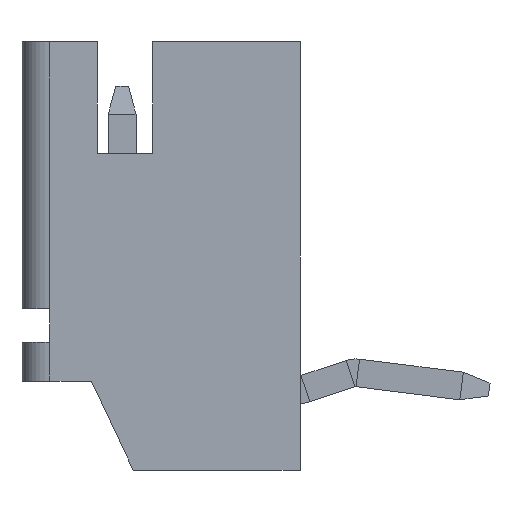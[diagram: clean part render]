
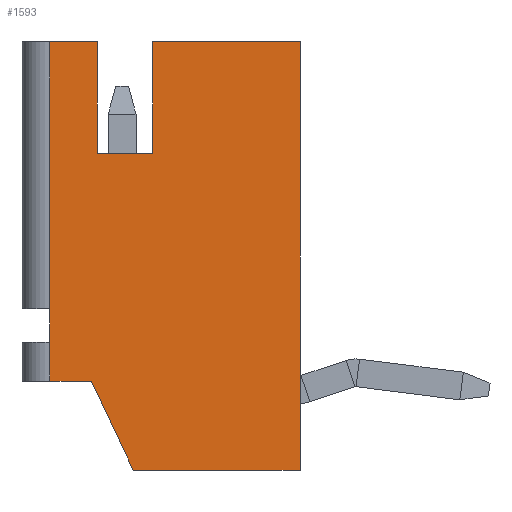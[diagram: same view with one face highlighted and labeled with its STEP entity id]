
A CAD part, left-side view. The second image highlights one B-rep face of the part: STEP entity #1593.
In plain terms, the highlighted planar face has unit normal (-1, 0, 0).
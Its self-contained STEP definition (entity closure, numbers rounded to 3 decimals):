
#33 = VERTEX_POINT ( 'NONE', #2794 ) ;
#44 = DIRECTION ( 'NONE',  ( 0., 0., -1. ) ) ;
#70 = EDGE_CURVE ( 'NONE', #2506, #1294, #556, .T. ) ;
#76 = VERTEX_POINT ( 'NONE', #2383 ) ;
#103 = CARTESIAN_POINT ( 'NONE',  ( -2., -3.2, 6.1 ) ) ;
#114 = LINE ( 'NONE', #1688, #1671 ) ;
#117 = DIRECTION ( 'NONE',  ( 0., 1., 0. ) ) ;
#133 = ORIENTED_EDGE ( 'NONE', *, *, #1596, .T. ) ;
#193 = CARTESIAN_POINT ( 'NONE',  ( -2., 1.8, 6.1 ) ) ;
#262 = LINE ( 'NONE', #103, #3092 ) ;
#361 = LINE ( 'NONE', #2526, #1074 ) ;
#376 = VERTEX_POINT ( 'NONE', #3053 ) ;
#392 = ORIENTED_EDGE ( 'NONE', *, *, #2105, .T. ) ;
#419 = EDGE_LOOP ( 'NONE', ( #2716, #1127, #1487, #392, #2181, #2623, #1104, #2550, #133, #2168, #3218, #2183 ) ) ;
#467 = VERTEX_POINT ( 'NONE', #1824 ) ;
#556 = LINE ( 'NONE', #812, #2613 ) ;
#565 = CARTESIAN_POINT ( 'NONE',  ( -2., 1.3, 0. ) ) ;
#611 = LINE ( 'NONE', #1985, #947 ) ;
#645 = CARTESIAN_POINT ( 'NONE',  ( -2., 1.3, 1.3 ) ) ;
#706 = VERTEX_POINT ( 'NONE', #565 ) ;
#744 = DIRECTION ( 'NONE',  ( 0., -0.424, -0.905 ) ) ;
#746 = VECTOR ( 'NONE', #2754, 1000. ) ;
#765 = EDGE_CURVE ( 'NONE', #467, #2108, #262, .T. ) ;
#770 = DIRECTION ( 'NONE',  ( 0., 0., 1. ) ) ;
#784 = DIRECTION ( 'NONE',  ( 0., 0., -1. ) ) ;
#800 = VECTOR ( 'NONE', #1504, 1000. ) ;
#812 = CARTESIAN_POINT ( 'NONE',  ( -2., 1.3, 1.3 ) ) ;
#815 = VERTEX_POINT ( 'NONE', #1666 ) ;
#823 = VECTOR ( 'NONE', #770, 1000. ) ;
#937 = EDGE_CURVE ( 'NONE', #33, #2583, #950, .T. ) ;
#942 = PLANE ( 'NONE',  #1615 ) ;
#947 = VECTOR ( 'NONE', #2175, 1000. ) ;
#950 = LINE ( 'NONE', #2002, #746 ) ;
#963 = CARTESIAN_POINT ( 'NONE',  ( -2., -0.55, 4.1 ) ) ;
#969 = DIRECTION ( 'NONE',  ( 0., -1., 0. ) ) ;
#1052 = CARTESIAN_POINT ( 'NONE',  ( -2., 1.3, 0.7 ) ) ;
#1074 = VECTOR ( 'NONE', #3316, 1000. ) ;
#1104 = ORIENTED_EDGE ( 'NONE', *, *, #1489, .T. ) ;
#1105 = VERTEX_POINT ( 'NONE', #1781 ) ;
#1127 = ORIENTED_EDGE ( 'NONE', *, *, #1295, .T. ) ;
#1146 = EDGE_CURVE ( 'NONE', #376, #2506, #361, .T. ) ;
#1284 = VECTOR ( 'NONE', #744, 1000. ) ;
#1294 = VERTEX_POINT ( 'NONE', #1052 ) ;
#1295 = EDGE_CURVE ( 'NONE', #1294, #706, #2111, .T. ) ;
#1316 = LINE ( 'NONE', #2077, #823 ) ;
#1358 = FACE_OUTER_BOUND ( 'NONE', #419, .T. ) ;
#1427 = CARTESIAN_POINT ( 'NONE',  ( -2., 0.45, 4.1 ) ) ;
#1487 = ORIENTED_EDGE ( 'NONE', *, *, #1996, .T. ) ;
#1489 = EDGE_CURVE ( 'NONE', #2108, #33, #114, .T. ) ;
#1504 = DIRECTION ( 'NONE',  ( 0., 1., 0. ) ) ;
#1553 = EDGE_CURVE ( 'NONE', #815, #467, #611, .T. ) ;
#1593 = ADVANCED_FACE ( 'NONE', ( #1358 ), #942, .T. ) ;
#1596 = EDGE_CURVE ( 'NONE', #2583, #76, #2187, .T. ) ;
#1615 = AXIS2_PLACEMENT_3D ( 'NONE', #2731, #2699, #1723 ) ;
#1645 = VECTOR ( 'NONE', #784, 1000. ) ;
#1666 = CARTESIAN_POINT ( 'NONE',  ( -2., -0.2, -1.6 ) ) ;
#1671 = VECTOR ( 'NONE', #117, 1000. ) ;
#1688 = CARTESIAN_POINT ( 'NONE',  ( -2., -0.55, 6.1 ) ) ;
#1717 = EDGE_CURVE ( 'NONE', #76, #3341, #1316, .T. ) ;
#1723 = DIRECTION ( 'NONE',  ( 0., -1., 0. ) ) ;
#1781 = CARTESIAN_POINT ( 'NONE',  ( -2., 0.55, 0. ) ) ;
#1824 = CARTESIAN_POINT ( 'NONE',  ( -2., -3.2, -1.6 ) ) ;
#1854 = CARTESIAN_POINT ( 'NONE',  ( -2., 1.3, 0. ) ) ;
#1985 = CARTESIAN_POINT ( 'NONE',  ( -2., -3.2, -1.6 ) ) ;
#1996 = EDGE_CURVE ( 'NONE', #706, #1105, #2745, .T. ) ;
#2002 = CARTESIAN_POINT ( 'NONE',  ( -2., -0.55, 6.1 ) ) ;
#2073 = VECTOR ( 'NONE', #2185, 1000. ) ;
#2077 = CARTESIAN_POINT ( 'NONE',  ( -2., 0.45, 6.1 ) ) ;
#2105 = EDGE_CURVE ( 'NONE', #1105, #815, #2557, .T. ) ;
#2108 = VERTEX_POINT ( 'NONE', #3259 ) ;
#2111 = LINE ( 'NONE', #1854, #1645 ) ;
#2168 = ORIENTED_EDGE ( 'NONE', *, *, #1717, .T. ) ;
#2175 = DIRECTION ( 'NONE',  ( 0., -1., 0. ) ) ;
#2181 = ORIENTED_EDGE ( 'NONE', *, *, #1553, .T. ) ;
#2183 = ORIENTED_EDGE ( 'NONE', *, *, #1146, .T. ) ;
#2185 = DIRECTION ( 'NONE',  ( 0., 1., 0. ) ) ;
#2187 = LINE ( 'NONE', #1427, #2073 ) ;
#2383 = CARTESIAN_POINT ( 'NONE',  ( -2., 0.45, 4.1 ) ) ;
#2440 = DIRECTION ( 'NONE',  ( 0., 0., 1. ) ) ;
#2479 = CARTESIAN_POINT ( 'NONE',  ( -2., 0.45, 6.1 ) ) ;
#2502 = CARTESIAN_POINT ( 'NONE',  ( -2., 1.8, 0. ) ) ;
#2506 = VERTEX_POINT ( 'NONE', #645 ) ;
#2526 = CARTESIAN_POINT ( 'NONE',  ( -2., 1.3, 0. ) ) ;
#2535 = CARTESIAN_POINT ( 'NONE',  ( -2., -0.2, -1.6 ) ) ;
#2550 = ORIENTED_EDGE ( 'NONE', *, *, #937, .T. ) ;
#2557 = LINE ( 'NONE', #2535, #1284 ) ;
#2583 = VERTEX_POINT ( 'NONE', #963 ) ;
#2613 = VECTOR ( 'NONE', #44, 1000. ) ;
#2623 = ORIENTED_EDGE ( 'NONE', *, *, #765, .T. ) ;
#2624 = VECTOR ( 'NONE', #969, 1000. ) ;
#2699 = DIRECTION ( 'NONE',  ( -1., 0., 0. ) ) ;
#2716 = ORIENTED_EDGE ( 'NONE', *, *, #70, .T. ) ;
#2731 = CARTESIAN_POINT ( 'NONE',  ( -2., 0., 0. ) ) ;
#2745 = LINE ( 'NONE', #2502, #2624 ) ;
#2754 = DIRECTION ( 'NONE',  ( 0., 0., -1. ) ) ;
#2781 = EDGE_CURVE ( 'NONE', #3341, #376, #3005, .T. ) ;
#2794 = CARTESIAN_POINT ( 'NONE',  ( -2., -0.55, 6.1 ) ) ;
#3005 = LINE ( 'NONE', #193, #800 ) ;
#3053 = CARTESIAN_POINT ( 'NONE',  ( -2., 1.3, 6.1 ) ) ;
#3092 = VECTOR ( 'NONE', #2440, 1000. ) ;
#3218 = ORIENTED_EDGE ( 'NONE', *, *, #2781, .T. ) ;
#3259 = CARTESIAN_POINT ( 'NONE',  ( -2., -3.2, 6.1 ) ) ;
#3316 = DIRECTION ( 'NONE',  ( 0., 0., -1. ) ) ;
#3341 = VERTEX_POINT ( 'NONE', #2479 ) ;
